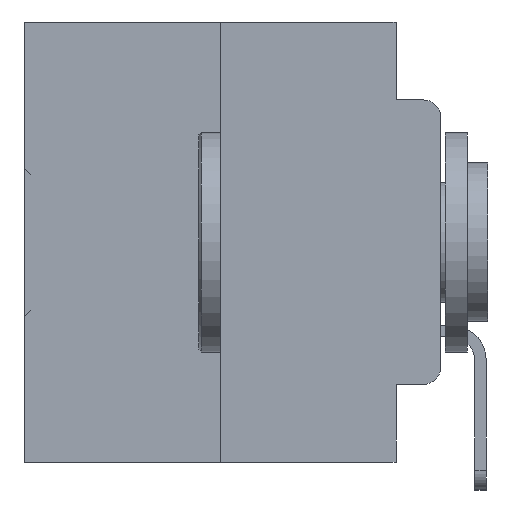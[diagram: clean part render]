
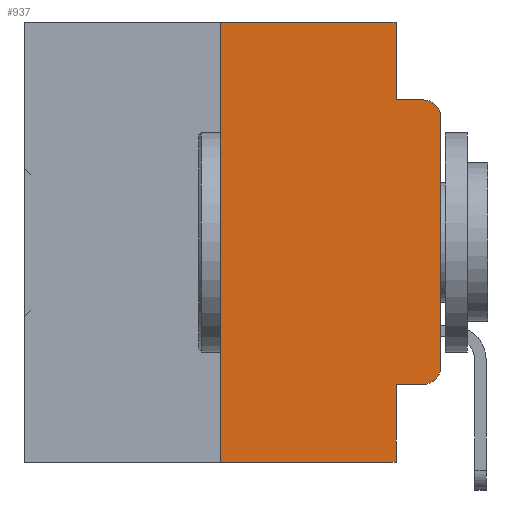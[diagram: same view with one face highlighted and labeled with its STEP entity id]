
A CAD part, left-side view. The second image highlights one B-rep face of the part: STEP entity #937.
In plain terms, the highlighted planar face has unit normal (-1, 0, 0).
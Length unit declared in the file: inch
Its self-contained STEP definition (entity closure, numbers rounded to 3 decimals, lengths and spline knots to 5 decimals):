
#360 = ORIENTED_EDGE ( 'NONE', *, *, #19779, .F. ) ;
#604 = EDGE_CURVE ( 'NONE', #21498, #1878, #21959, .T. ) ;
#728 = DIRECTION ( 'NONE',  ( 0., -1., 0. ) ) ;
#937 = ADVANCED_FACE ( 'NONE', ( #4773 ), #16264, .F. ) ;
#1212 = LINE ( 'NONE', #5553, #8262 ) ;
#1580 = ORIENTED_EDGE ( 'NONE', *, *, #25146, .T. ) ;
#1878 = VERTEX_POINT ( 'NONE', #13275 ) ;
#2025 = VERTEX_POINT ( 'NONE', #21767 ) ;
#2158 = DIRECTION ( 'NONE',  ( 0., 0., -1. ) ) ;
#2206 = DIRECTION ( 'NONE',  ( 1., 0., 0. ) ) ;
#2558 = EDGE_CURVE ( 'NONE', #24926, #21498, #31651, .T. ) ;
#3217 = VECTOR ( 'NONE', #728, 39.37008 ) ;
#3512 = ORIENTED_EDGE ( 'NONE', *, *, #18024, .F. ) ;
#3717 = VERTEX_POINT ( 'NONE', #6414 ) ;
#4314 = AXIS2_PLACEMENT_3D ( 'NONE', #16267, #2206, #2158 ) ;
#4583 = EDGE_CURVE ( 'NONE', #24926, #3717, #7216, .T. ) ;
#4773 = FACE_OUTER_BOUND ( 'NONE', #25982, .T. ) ;
#4826 = ORIENTED_EDGE ( 'NONE', *, *, #21573, .T. ) ;
#5553 = CARTESIAN_POINT ( 'NONE',  ( 0., 0.473, -0.5 ) ) ;
#6414 = CARTESIAN_POINT ( 'NONE',  ( 0., 0.051, -0.5 ) ) ;
#6440 = LINE ( 'NONE', #20883, #20480 ) ;
#6588 = EDGE_CURVE ( 'NONE', #14261, #16767, #33066, .T. ) ;
#6907 = CARTESIAN_POINT ( 'NONE',  ( 0., 0.25, 0. ) ) ;
#7087 = AXIS2_PLACEMENT_3D ( 'NONE', #29150, #29147, #29075 ) ;
#7216 = LINE ( 'NONE', #33907, #35004 ) ;
#7310 = VERTEX_POINT ( 'NONE', #32343 ) ;
#7415 = AXIS2_PLACEMENT_3D ( 'NONE', #28348, #12327, #30932 ) ;
#8262 = VECTOR ( 'NONE', #30258, 39.37008 ) ;
#8344 = CARTESIAN_POINT ( 'NONE',  ( 0., 0., 0. ) ) ;
#8986 = CARTESIAN_POINT ( 'NONE',  ( 0., 0.02, -0.4115 ) ) ;
#9064 = CARTESIAN_POINT ( 'NONE',  ( 0., 0.02, -0.0885 ) ) ;
#9527 = ORIENTED_EDGE ( 'NONE', *, *, #27347, .T. ) ;
#9649 = VECTOR ( 'NONE', #34794, 39.37008 ) ;
#9962 = LINE ( 'NONE', #14294, #10889 ) ;
#9985 = DIRECTION ( 'NONE',  ( 0., 0., -1. ) ) ;
#10735 = CARTESIAN_POINT ( 'NONE',  ( 0., 0.25, 0. ) ) ;
#10889 = VECTOR ( 'NONE', #24957, 39.37008 ) ;
#12327 = DIRECTION ( 'NONE',  ( -1., 0., 0. ) ) ;
#12587 = CIRCLE ( 'NONE', #7415, 0.02 ) ;
#12807 = VECTOR ( 'NONE', #26192, 39.37008 ) ;
#13271 = ORIENTED_EDGE ( 'NONE', *, *, #6588, .F. ) ;
#13275 = CARTESIAN_POINT ( 'NONE',  ( 0., 0., -0.3915 ) ) ;
#14261 = VERTEX_POINT ( 'NONE', #22907 ) ;
#14294 = CARTESIAN_POINT ( 'NONE',  ( 0., 0.473, 0. ) ) ;
#16053 = CARTESIAN_POINT ( 'NONE',  ( 0., 0.051, -0.4115 ) ) ;
#16264 = PLANE ( 'NONE',  #4314 ) ;
#16267 = CARTESIAN_POINT ( 'NONE',  ( 0., 0.473, 0. ) ) ;
#16767 = VERTEX_POINT ( 'NONE', #10735 ) ;
#16928 = EDGE_CURVE ( 'NONE', #16767, #7310, #9962, .T. ) ;
#17180 = ORIENTED_EDGE ( 'NONE', *, *, #4583, .F. ) ;
#17642 = ORIENTED_EDGE ( 'NONE', *, *, #604, .T. ) ;
#17942 = LINE ( 'NONE', #32234, #9649 ) ;
#18024 = EDGE_CURVE ( 'NONE', #7310, #32706, #6440, .T. ) ;
#18212 = ORIENTED_EDGE ( 'NONE', *, *, #2558, .T. ) ;
#18374 = ORIENTED_EDGE ( 'NONE', *, *, #16928, .F. ) ;
#19779 = EDGE_CURVE ( 'NONE', #32706, #20210, #17942, .T. ) ;
#20210 = VERTEX_POINT ( 'NONE', #9064 ) ;
#20480 = VECTOR ( 'NONE', #28958, 39.37008 ) ;
#20688 = CARTESIAN_POINT ( 'NONE',  ( 0., 0.051, -0.0885 ) ) ;
#20883 = CARTESIAN_POINT ( 'NONE',  ( 0., 0.051, 0. ) ) ;
#21498 = VERTEX_POINT ( 'NONE', #8986 ) ;
#21573 = EDGE_CURVE ( 'NONE', #2025, #20210, #12587, .T. ) ;
#21767 = CARTESIAN_POINT ( 'NONE',  ( 0., 0., -0.1085 ) ) ;
#21959 = CIRCLE ( 'NONE', #7087, 0.02 ) ;
#22907 = CARTESIAN_POINT ( 'NONE',  ( 0., 0.25, -0.5 ) ) ;
#23770 = CARTESIAN_POINT ( 'NONE',  ( 0., 0.051, -0.4115 ) ) ;
#24772 = DIRECTION ( 'NONE',  ( 0., 0., 1. ) ) ;
#24926 = VERTEX_POINT ( 'NONE', #23770 ) ;
#24957 = DIRECTION ( 'NONE',  ( 0., -1., 0. ) ) ;
#25146 = EDGE_CURVE ( 'NONE', #1878, #2025, #28413, .T. ) ;
#25982 = EDGE_LOOP ( 'NONE', ( #1580, #4826, #360, #3512, #18374, #13271, #9527, #17180, #18212, #17642 ) ) ;
#26192 = DIRECTION ( 'NONE',  ( 0., 0., 1. ) ) ;
#26792 = VECTOR ( 'NONE', #24772, 39.37008 ) ;
#27347 = EDGE_CURVE ( 'NONE', #14261, #3717, #1212, .T. ) ;
#28348 = CARTESIAN_POINT ( 'NONE',  ( 0., 0.02, -0.1085 ) ) ;
#28413 = LINE ( 'NONE', #8344, #26792 ) ;
#28958 = DIRECTION ( 'NONE',  ( 0., 0., -1. ) ) ;
#29075 = DIRECTION ( 'NONE',  ( 0., 0., -1. ) ) ;
#29147 = DIRECTION ( 'NONE',  ( -1., 0., 0. ) ) ;
#29150 = CARTESIAN_POINT ( 'NONE',  ( 0., 0.02, -0.3915 ) ) ;
#30258 = DIRECTION ( 'NONE',  ( 0., -1., 0. ) ) ;
#30932 = DIRECTION ( 'NONE',  ( 0., 0., -1. ) ) ;
#31651 = LINE ( 'NONE', #16053, #3217 ) ;
#32234 = CARTESIAN_POINT ( 'NONE',  ( 0., 0.051, -0.0885 ) ) ;
#32343 = CARTESIAN_POINT ( 'NONE',  ( 0., 0.051, 0. ) ) ;
#32706 = VERTEX_POINT ( 'NONE', #20688 ) ;
#33066 = LINE ( 'NONE', #6907, #12807 ) ;
#33907 = CARTESIAN_POINT ( 'NONE',  ( 0., 0.051, 0. ) ) ;
#34794 = DIRECTION ( 'NONE',  ( 0., -1., 0. ) ) ;
#35004 = VECTOR ( 'NONE', #9985, 39.37008 ) ;
